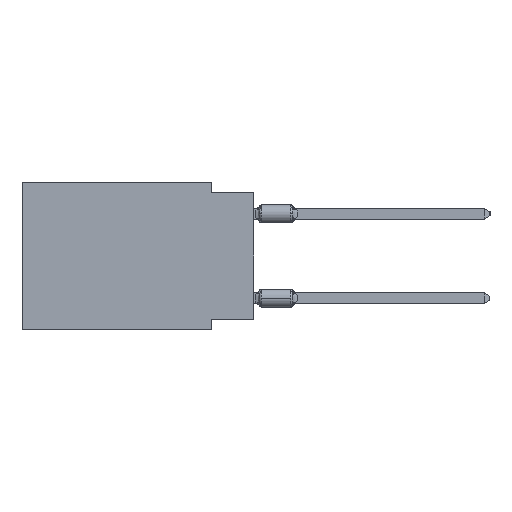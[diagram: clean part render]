
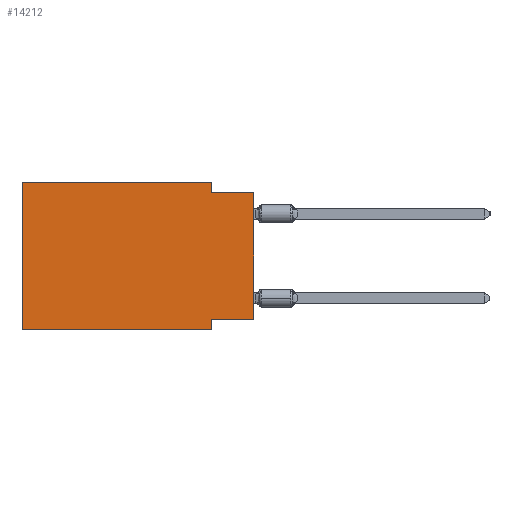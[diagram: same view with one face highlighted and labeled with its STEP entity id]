
A CAD part, left-side view. The second image highlights one B-rep face of the part: STEP entity #14212.
In plain terms, the highlighted planar face has unit normal (-1, 0, 0).
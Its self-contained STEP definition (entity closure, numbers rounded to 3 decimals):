
#656 = DIRECTION ( 'NONE',  ( 1., 0., 0. ) ) ;
#1385 = VECTOR ( 'NONE', #5961, 1000. ) ;
#2026 = ORIENTED_EDGE ( 'NONE', *, *, #18787, .F. ) ;
#2199 = ORIENTED_EDGE ( 'NONE', *, *, #8510, .F. ) ;
#3037 = ORIENTED_EDGE ( 'NONE', *, *, #33025, .T. ) ;
#3048 = DIRECTION ( 'NONE',  ( 0., 0., -1. ) ) ;
#3651 = LINE ( 'NONE', #19902, #5559 ) ;
#3808 = ORIENTED_EDGE ( 'NONE', *, *, #30686, .F. ) ;
#3854 = LINE ( 'NONE', #9699, #36907 ) ;
#4164 = CARTESIAN_POINT ( 'NONE',  ( 0., 0., -8.255 ) ) ;
#4903 = LINE ( 'NONE', #14010, #28989 ) ;
#5530 = CARTESIAN_POINT ( 'NONE',  ( 0., 13.97, -8.89 ) ) ;
#5559 = VECTOR ( 'NONE', #26830, 1000. ) ;
#5961 = DIRECTION ( 'NONE',  ( 0., -1., 0. ) ) ;
#6055 = VERTEX_POINT ( 'NONE', #31354 ) ;
#6257 = VERTEX_POINT ( 'NONE', #42400 ) ;
#7377 = VECTOR ( 'NONE', #7654, 1000. ) ;
#7654 = DIRECTION ( 'NONE',  ( 0., -1., 0. ) ) ;
#7941 = EDGE_LOOP ( 'NONE', ( #3037, #38916, #40462, #2026, #30073, #41532, #2199, #3808 ) ) ;
#8510 = EDGE_CURVE ( 'NONE', #25906, #6257, #27167, .T. ) ;
#9699 = CARTESIAN_POINT ( 'NONE',  ( 0., 2.54, 0. ) ) ;
#10616 = PLANE ( 'NONE',  #13370 ) ;
#11284 = CARTESIAN_POINT ( 'NONE',  ( 0., 2.54, -8.255 ) ) ;
#11553 = DIRECTION ( 'NONE',  ( 0., 0., 1. ) ) ;
#11748 = VERTEX_POINT ( 'NONE', #4164 ) ;
#12577 = CARTESIAN_POINT ( 'NONE',  ( 0., 2.54, -0.635 ) ) ;
#13370 = AXIS2_PLACEMENT_3D ( 'NONE', #42711, #656, #3048 ) ;
#14010 = CARTESIAN_POINT ( 'NONE',  ( 0., 0., -0.635 ) ) ;
#14212 = ADVANCED_FACE ( 'NONE', ( #19941 ), #10616, .F. ) ;
#14682 = EDGE_CURVE ( 'NONE', #6055, #33160, #3854, .T. ) ;
#14812 = LINE ( 'NONE', #28011, #25887 ) ;
#18227 = CARTESIAN_POINT ( 'NONE',  ( 0., 0., 0. ) ) ;
#18787 = EDGE_CURVE ( 'NONE', #23289, #6055, #37331, .T. ) ;
#19902 = CARTESIAN_POINT ( 'NONE',  ( 0., 0., -8.255 ) ) ;
#19941 = FACE_OUTER_BOUND ( 'NONE', #7941, .T. ) ;
#20112 = DIRECTION ( 'NONE',  ( 0., 0., -1. ) ) ;
#20461 = DIRECTION ( 'NONE',  ( 0., 0., -1. ) ) ;
#22420 = LINE ( 'NONE', #5530, #1385 ) ;
#22707 = EDGE_CURVE ( 'NONE', #33160, #33692, #4903, .T. ) ;
#23289 = VERTEX_POINT ( 'NONE', #34503 ) ;
#23398 = VERTEX_POINT ( 'NONE', #42316 ) ;
#24064 = EDGE_CURVE ( 'NONE', #23398, #6257, #22420, .T. ) ;
#24716 = DIRECTION ( 'NONE',  ( 0., 0., 1. ) ) ;
#25887 = VECTOR ( 'NONE', #11553, 1000. ) ;
#25906 = VERTEX_POINT ( 'NONE', #11284 ) ;
#26830 = DIRECTION ( 'NONE',  ( 0., 1., 0. ) ) ;
#27167 = LINE ( 'NONE', #30837, #35922 ) ;
#27363 = CARTESIAN_POINT ( 'NONE',  ( 0., 13.97, 0. ) ) ;
#28011 = CARTESIAN_POINT ( 'NONE',  ( 0., 13.97, 0. ) ) ;
#28989 = VECTOR ( 'NONE', #37190, 1000. ) ;
#30073 = ORIENTED_EDGE ( 'NONE', *, *, #36662, .F. ) ;
#30686 = EDGE_CURVE ( 'NONE', #11748, #25906, #3651, .T. ) ;
#30837 = CARTESIAN_POINT ( 'NONE',  ( 0., 2.54, -8.89 ) ) ;
#31354 = CARTESIAN_POINT ( 'NONE',  ( 0., 2.54, 0. ) ) ;
#33025 = EDGE_CURVE ( 'NONE', #11748, #33692, #34678, .T. ) ;
#33160 = VERTEX_POINT ( 'NONE', #12577 ) ;
#33274 = VECTOR ( 'NONE', #24716, 1000. ) ;
#33692 = VERTEX_POINT ( 'NONE', #34298 ) ;
#34298 = CARTESIAN_POINT ( 'NONE',  ( 0., 0., -0.635 ) ) ;
#34503 = CARTESIAN_POINT ( 'NONE',  ( 0., 13.97, 0. ) ) ;
#34678 = LINE ( 'NONE', #18227, #33274 ) ;
#35922 = VECTOR ( 'NONE', #20461, 1000. ) ;
#36662 = EDGE_CURVE ( 'NONE', #23398, #23289, #14812, .T. ) ;
#36907 = VECTOR ( 'NONE', #20112, 1000. ) ;
#37190 = DIRECTION ( 'NONE',  ( 0., -1., 0. ) ) ;
#37331 = LINE ( 'NONE', #27363, #7377 ) ;
#38916 = ORIENTED_EDGE ( 'NONE', *, *, #22707, .F. ) ;
#40462 = ORIENTED_EDGE ( 'NONE', *, *, #14682, .F. ) ;
#41532 = ORIENTED_EDGE ( 'NONE', *, *, #24064, .T. ) ;
#42316 = CARTESIAN_POINT ( 'NONE',  ( 0., 13.97, -8.89 ) ) ;
#42400 = CARTESIAN_POINT ( 'NONE',  ( 0., 2.54, -8.89 ) ) ;
#42711 = CARTESIAN_POINT ( 'NONE',  ( 0., 13.97, 0. ) ) ;
